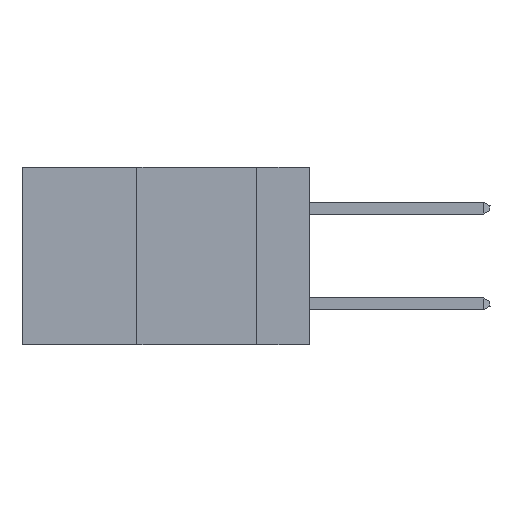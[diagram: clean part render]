
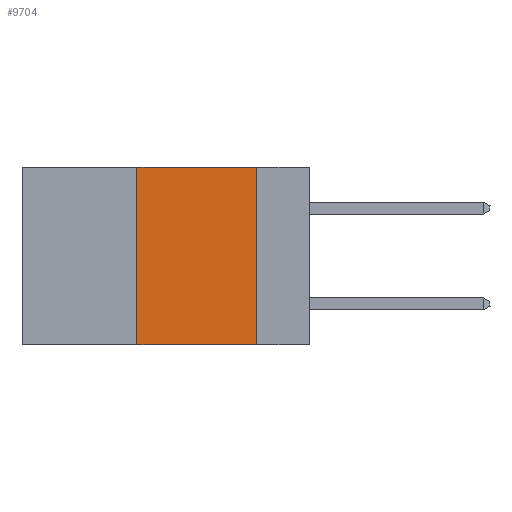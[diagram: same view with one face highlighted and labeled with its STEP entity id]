
A CAD part, left-side view. The second image highlights one B-rep face of the part: STEP entity #9704.
In plain terms, the highlighted planar face has unit normal (-1, 0, 0).
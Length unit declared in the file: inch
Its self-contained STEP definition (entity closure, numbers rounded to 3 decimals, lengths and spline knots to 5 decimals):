
#350 = VECTOR ( 'NONE', #28984, 39.37008 ) ;
#2324 = CARTESIAN_POINT ( 'NONE',  ( 0., 0.6, -0.37 ) ) ;
#4824 = DIRECTION ( 'NONE',  ( 0., 0., -1. ) ) ;
#7316 = CARTESIAN_POINT ( 'NONE',  ( 0., 0.6, 0. ) ) ;
#7479 = PLANE ( 'NONE',  #8441 ) ;
#8282 = EDGE_CURVE ( 'NONE', #43181, #12299, #13186, .T. ) ;
#8441 = AXIS2_PLACEMENT_3D ( 'NONE', #7316, #43962, #33044 ) ;
#9704 = ADVANCED_FACE ( 'NONE', ( #24444 ), #7479, .F. ) ;
#12299 = VERTEX_POINT ( 'NONE', #15029 ) ;
#13186 = LINE ( 'NONE', #13720, #37735 ) ;
#13720 = CARTESIAN_POINT ( 'NONE',  ( 0., 0.6, 0. ) ) ;
#15029 = CARTESIAN_POINT ( 'NONE',  ( 0., 0.11, 0. ) ) ;
#16861 = ORIENTED_EDGE ( 'NONE', *, *, #8282, .F. ) ;
#17189 = CARTESIAN_POINT ( 'NONE',  ( 0., 0.36, -0.37 ) ) ;
#17401 = ORIENTED_EDGE ( 'NONE', *, *, #34069, .T. ) ;
#17518 = DIRECTION ( 'NONE',  ( 0., -1., 0. ) ) ;
#22232 = VECTOR ( 'NONE', #38087, 39.37008 ) ;
#23427 = EDGE_CURVE ( 'NONE', #12299, #37230, #38922, .T. ) ;
#24444 = FACE_OUTER_BOUND ( 'NONE', #28683, .T. ) ;
#24457 = VERTEX_POINT ( 'NONE', #17189 ) ;
#27169 = CARTESIAN_POINT ( 'NONE',  ( 0., 0.36, 0. ) ) ;
#28683 = EDGE_LOOP ( 'NONE', ( #39606, #16861, #46851, #17401 ) ) ;
#28984 = DIRECTION ( 'NONE',  ( 0., -1., 0. ) ) ;
#30547 = CARTESIAN_POINT ( 'NONE',  ( 0., 0.11, 0. ) ) ;
#32195 = CARTESIAN_POINT ( 'NONE',  ( 0., 0.36, 0. ) ) ;
#33044 = DIRECTION ( 'NONE',  ( 0., 0., -1. ) ) ;
#33517 = LINE ( 'NONE', #2324, #350 ) ;
#34069 = EDGE_CURVE ( 'NONE', #24457, #37230, #33517, .T. ) ;
#37230 = VERTEX_POINT ( 'NONE', #42614 ) ;
#37735 = VECTOR ( 'NONE', #17518, 39.37008 ) ;
#38087 = DIRECTION ( 'NONE',  ( 0., 0., 1. ) ) ;
#38922 = LINE ( 'NONE', #30547, #40091 ) ;
#39606 = ORIENTED_EDGE ( 'NONE', *, *, #23427, .F. ) ;
#40091 = VECTOR ( 'NONE', #4824, 39.37008 ) ;
#40146 = EDGE_CURVE ( 'NONE', #24457, #43181, #42857, .T. ) ;
#42614 = CARTESIAN_POINT ( 'NONE',  ( 0., 0.11, -0.37 ) ) ;
#42857 = LINE ( 'NONE', #27169, #22232 ) ;
#43181 = VERTEX_POINT ( 'NONE', #32195 ) ;
#43962 = DIRECTION ( 'NONE',  ( 1., 0., 0. ) ) ;
#46851 = ORIENTED_EDGE ( 'NONE', *, *, #40146, .F. ) ;
